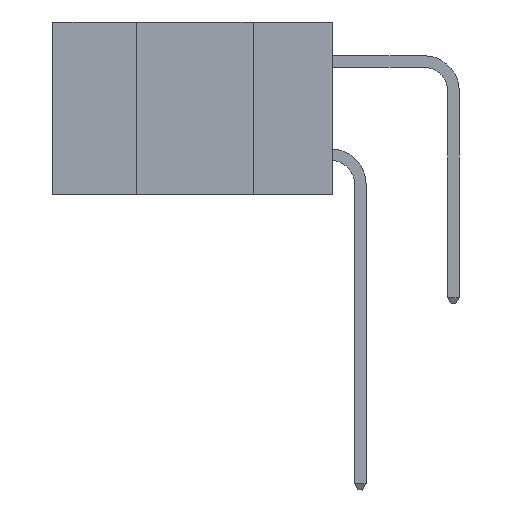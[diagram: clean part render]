
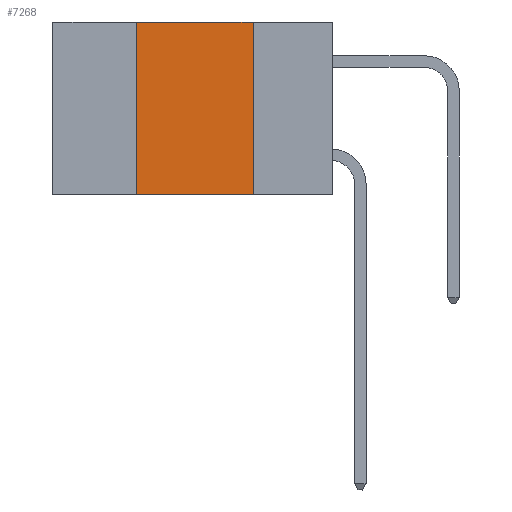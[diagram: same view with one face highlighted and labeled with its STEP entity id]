
A CAD part, left-side view. The second image highlights one B-rep face of the part: STEP entity #7268.
In plain terms, the highlighted planar face has unit normal (-1, 0, 0).
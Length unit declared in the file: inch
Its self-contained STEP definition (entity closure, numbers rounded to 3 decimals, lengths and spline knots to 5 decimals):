
#150 = VECTOR ( 'NONE', #25159, 39.37008 ) ;
#874 = ORIENTED_EDGE ( 'NONE', *, *, #3410, .F. ) ;
#1121 = VERTEX_POINT ( 'NONE', #25293 ) ;
#1681 = EDGE_CURVE ( 'NONE', #18792, #2632, #25010, .T. ) ;
#1862 = VECTOR ( 'NONE', #8728, 39.37008 ) ;
#2537 = CARTESIAN_POINT ( 'NONE',  ( 0., 0.17, 0. ) ) ;
#2632 = VERTEX_POINT ( 'NONE', #2537 ) ;
#2725 = CARTESIAN_POINT ( 'NONE',  ( 0., 0.6, -0.37 ) ) ;
#3212 = LINE ( 'NONE', #18795, #1862 ) ;
#3410 = EDGE_CURVE ( 'NONE', #1121, #18792, #16059, .T. ) ;
#3985 = VERTEX_POINT ( 'NONE', #13858 ) ;
#6534 = ORIENTED_EDGE ( 'NONE', *, *, #7654, .T. ) ;
#7268 = ADVANCED_FACE ( 'NONE', ( #9402 ), #22208, .F. ) ;
#7654 = EDGE_CURVE ( 'NONE', #1121, #3985, #16673, .T. ) ;
#8013 = CARTESIAN_POINT ( 'NONE',  ( 0., 0.6, 0. ) ) ;
#8728 = DIRECTION ( 'NONE',  ( 0., 0., -1. ) ) ;
#9402 = FACE_OUTER_BOUND ( 'NONE', #23590, .T. ) ;
#10633 = VECTOR ( 'NONE', #25107, 39.37008 ) ;
#12085 = DIRECTION ( 'NONE',  ( 0., 0., -1. ) ) ;
#13128 = EDGE_CURVE ( 'NONE', #2632, #3985, #3212, .T. ) ;
#13858 = CARTESIAN_POINT ( 'NONE',  ( 0., 0.17, -0.37 ) ) ;
#16059 = LINE ( 'NONE', #25653, #10633 ) ;
#16089 = ORIENTED_EDGE ( 'NONE', *, *, #1681, .F. ) ;
#16673 = LINE ( 'NONE', #2725, #150 ) ;
#18730 = CARTESIAN_POINT ( 'NONE',  ( 0., 0.42, 0. ) ) ;
#18792 = VERTEX_POINT ( 'NONE', #18730 ) ;
#18795 = CARTESIAN_POINT ( 'NONE',  ( 0., 0.17, 0. ) ) ;
#19610 = VECTOR ( 'NONE', #24838, 39.37008 ) ;
#20156 = ORIENTED_EDGE ( 'NONE', *, *, #13128, .F. ) ;
#20502 = CARTESIAN_POINT ( 'NONE',  ( 0., 0.6, 0. ) ) ;
#22208 = PLANE ( 'NONE',  #25425 ) ;
#23590 = EDGE_LOOP ( 'NONE', ( #20156, #16089, #874, #6534 ) ) ;
#24212 = DIRECTION ( 'NONE',  ( 1., 0., 0. ) ) ;
#24838 = DIRECTION ( 'NONE',  ( 0., -1., 0. ) ) ;
#25010 = LINE ( 'NONE', #20502, #19610 ) ;
#25107 = DIRECTION ( 'NONE',  ( 0., 0., 1. ) ) ;
#25159 = DIRECTION ( 'NONE',  ( 0., -1., 0. ) ) ;
#25293 = CARTESIAN_POINT ( 'NONE',  ( 0., 0.42, -0.37 ) ) ;
#25425 = AXIS2_PLACEMENT_3D ( 'NONE', #8013, #24212, #12085 ) ;
#25653 = CARTESIAN_POINT ( 'NONE',  ( 0., 0.42, 0. ) ) ;
